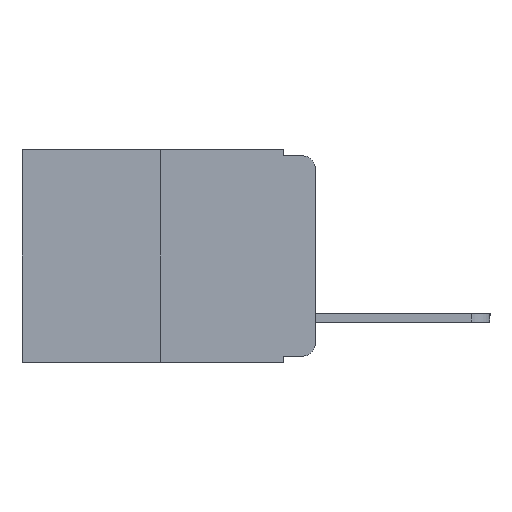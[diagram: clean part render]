
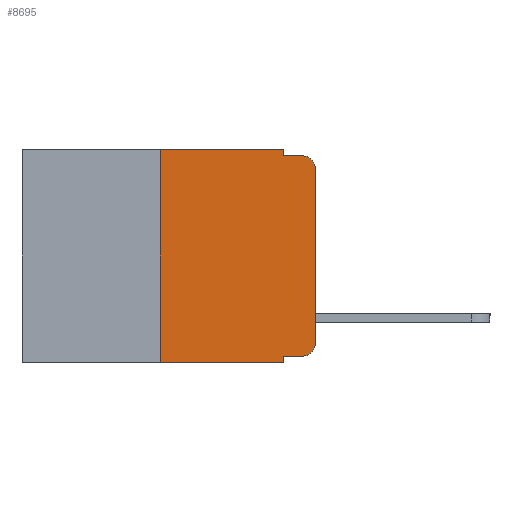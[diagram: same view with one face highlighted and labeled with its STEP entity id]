
A CAD part, left-side view. The second image highlights one B-rep face of the part: STEP entity #8695.
In plain terms, the highlighted planar face has unit normal (-1, 0, 0).
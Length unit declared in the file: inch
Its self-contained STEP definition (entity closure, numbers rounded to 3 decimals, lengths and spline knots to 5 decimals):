
#16 = CARTESIAN_POINT ( 'NONE',  ( 0., 0., 0. ) ) ;
#366 = VERTEX_POINT ( 'NONE', #7535 ) ;
#466 = ORIENTED_EDGE ( 'NONE', *, *, #8362, .F. ) ;
#782 = ORIENTED_EDGE ( 'NONE', *, *, #7719, .T. ) ;
#792 = CARTESIAN_POINT ( 'NONE',  ( 0., 0.473, -0.343 ) ) ;
#828 = LINE ( 'NONE', #9712, #11036 ) ;
#1120 = ORIENTED_EDGE ( 'NONE', *, *, #8905, .T. ) ;
#1140 = DIRECTION ( 'NONE',  ( 0., 0., -1. ) ) ;
#1165 = ORIENTED_EDGE ( 'NONE', *, *, #8487, .F. ) ;
#1185 = ORIENTED_EDGE ( 'NONE', *, *, #7578, .T. ) ;
#1192 = CARTESIAN_POINT ( 'NONE',  ( 0., 0.25, 0. ) ) ;
#1209 = EDGE_LOOP ( 'NONE', ( #1185, #782, #466, #1165, #6579, #2946, #6162, #6950, #7418, #1120 ) ) ;
#1513 = CARTESIAN_POINT ( 'NONE',  ( 0., 0.473, 0. ) ) ;
#1600 = VECTOR ( 'NONE', #1140, 39.37008 ) ;
#1645 = CARTESIAN_POINT ( 'NONE',  ( 0., 0.02, -0.01 ) ) ;
#1741 = VERTEX_POINT ( 'NONE', #7882 ) ;
#1817 = VERTEX_POINT ( 'NONE', #3651 ) ;
#1884 = DIRECTION ( 'NONE',  ( 0., -1., 0. ) ) ;
#1897 = VERTEX_POINT ( 'NONE', #6468 ) ;
#1902 = CARTESIAN_POINT ( 'NONE',  ( 0., 0.051, 0. ) ) ;
#2307 = CARTESIAN_POINT ( 'NONE',  ( 0., 0.473, 0. ) ) ;
#2565 = PLANE ( 'NONE',  #2915 ) ;
#2582 = LINE ( 'NONE', #12277, #7293 ) ;
#2751 = AXIS2_PLACEMENT_3D ( 'NONE', #6085, #12382, #7048 ) ;
#2915 = AXIS2_PLACEMENT_3D ( 'NONE', #1513, #10373, #4695 ) ;
#2946 = ORIENTED_EDGE ( 'NONE', *, *, #8529, .F. ) ;
#3137 = VERTEX_POINT ( 'NONE', #11795 ) ;
#3381 = AXIS2_PLACEMENT_3D ( 'NONE', #6025, #12332, #6985 ) ;
#3624 = VECTOR ( 'NONE', #7969, 39.37008 ) ;
#3651 = CARTESIAN_POINT ( 'NONE',  ( 0., 0., -0.03 ) ) ;
#4440 = VERTEX_POINT ( 'NONE', #9801 ) ;
#4695 = DIRECTION ( 'NONE',  ( 0., 0., -1. ) ) ;
#4917 = VERTEX_POINT ( 'NONE', #10758 ) ;
#4977 = CARTESIAN_POINT ( 'NONE',  ( 0., 0.051, -0.333 ) ) ;
#5390 = VERTEX_POINT ( 'NONE', #1645 ) ;
#5427 = DIRECTION ( 'NONE',  ( 0., 0., 1. ) ) ;
#5476 = VECTOR ( 'NONE', #6401, 39.37008 ) ;
#5544 = EDGE_CURVE ( 'NONE', #7499, #3137, #8556, .T. ) ;
#5793 = LINE ( 'NONE', #2307, #10792 ) ;
#5956 = DIRECTION ( 'NONE',  ( 0., -1., 0. ) ) ;
#6025 = CARTESIAN_POINT ( 'NONE',  ( 0., 0.02, -0.03 ) ) ;
#6079 = VECTOR ( 'NONE', #5956, 39.37008 ) ;
#6085 = CARTESIAN_POINT ( 'NONE',  ( 0., 0.02, -0.313 ) ) ;
#6162 = ORIENTED_EDGE ( 'NONE', *, *, #5544, .T. ) ;
#6401 = DIRECTION ( 'NONE',  ( 0., 0., 1. ) ) ;
#6468 = CARTESIAN_POINT ( 'NONE',  ( 0., 0.02, -0.333 ) ) ;
#6579 = ORIENTED_EDGE ( 'NONE', *, *, #8520, .F. ) ;
#6950 = ORIENTED_EDGE ( 'NONE', *, *, #8845, .F. ) ;
#6985 = DIRECTION ( 'NONE',  ( 0., 0., -1. ) ) ;
#7048 = DIRECTION ( 'NONE',  ( 0., 0., -1. ) ) ;
#7293 = VECTOR ( 'NONE', #1884, 39.37008 ) ;
#7418 = ORIENTED_EDGE ( 'NONE', *, *, #8848, .T. ) ;
#7445 = LINE ( 'NONE', #16, #11921 ) ;
#7499 = VERTEX_POINT ( 'NONE', #12560 ) ;
#7535 = CARTESIAN_POINT ( 'NONE',  ( 0., 0., -0.313 ) ) ;
#7578 = EDGE_CURVE ( 'NONE', #366, #1817, #7445, .T. ) ;
#7719 = EDGE_CURVE ( 'NONE', #1817, #5390, #7899, .T. ) ;
#7882 = CARTESIAN_POINT ( 'NONE',  ( 0., 0.25, 0. ) ) ;
#7899 = CIRCLE ( 'NONE', #3381, 0.02 ) ;
#7969 = DIRECTION ( 'NONE',  ( 0., -1., 0. ) ) ;
#8054 = LINE ( 'NONE', #1192, #5476 ) ;
#8247 = CARTESIAN_POINT ( 'NONE',  ( 0., 0.051, 0. ) ) ;
#8362 = EDGE_CURVE ( 'NONE', #4440, #5390, #2582, .T. ) ;
#8487 = EDGE_CURVE ( 'NONE', #9534, #4440, #11046, .T. ) ;
#8520 = EDGE_CURVE ( 'NONE', #1741, #9534, #5793, .T. ) ;
#8529 = EDGE_CURVE ( 'NONE', #7499, #1741, #8054, .T. ) ;
#8556 = LINE ( 'NONE', #792, #3624 ) ;
#8695 = ADVANCED_FACE ( 'NONE', ( #8774 ), #2565, .F. ) ;
#8774 = FACE_OUTER_BOUND ( 'NONE', #1209, .T. ) ;
#8845 = EDGE_CURVE ( 'NONE', #4917, #3137, #828, .T. ) ;
#8848 = EDGE_CURVE ( 'NONE', #4917, #1897, #9217, .T. ) ;
#8905 = EDGE_CURVE ( 'NONE', #1897, #366, #12409, .T. ) ;
#9217 = LINE ( 'NONE', #4977, #6079 ) ;
#9220 = DIRECTION ( 'NONE',  ( 0., -1., 0. ) ) ;
#9534 = VERTEX_POINT ( 'NONE', #1902 ) ;
#9712 = CARTESIAN_POINT ( 'NONE',  ( 0., 0.051, 0. ) ) ;
#9801 = CARTESIAN_POINT ( 'NONE',  ( 0., 0.051, -0.01 ) ) ;
#10373 = DIRECTION ( 'NONE',  ( 1., 0., 0. ) ) ;
#10637 = DIRECTION ( 'NONE',  ( 0., 0., -1. ) ) ;
#10758 = CARTESIAN_POINT ( 'NONE',  ( 0., 0.051, -0.333 ) ) ;
#10792 = VECTOR ( 'NONE', #9220, 39.37008 ) ;
#11036 = VECTOR ( 'NONE', #10637, 39.37008 ) ;
#11046 = LINE ( 'NONE', #8247, #1600 ) ;
#11795 = CARTESIAN_POINT ( 'NONE',  ( 0., 0.051, -0.343 ) ) ;
#11921 = VECTOR ( 'NONE', #5427, 39.37008 ) ;
#12277 = CARTESIAN_POINT ( 'NONE',  ( 0., 0.051, -0.01 ) ) ;
#12332 = DIRECTION ( 'NONE',  ( -1., 0., 0. ) ) ;
#12382 = DIRECTION ( 'NONE',  ( -1., 0., 0. ) ) ;
#12409 = CIRCLE ( 'NONE', #2751, 0.02 ) ;
#12560 = CARTESIAN_POINT ( 'NONE',  ( 0., 0.25, -0.343 ) ) ;
